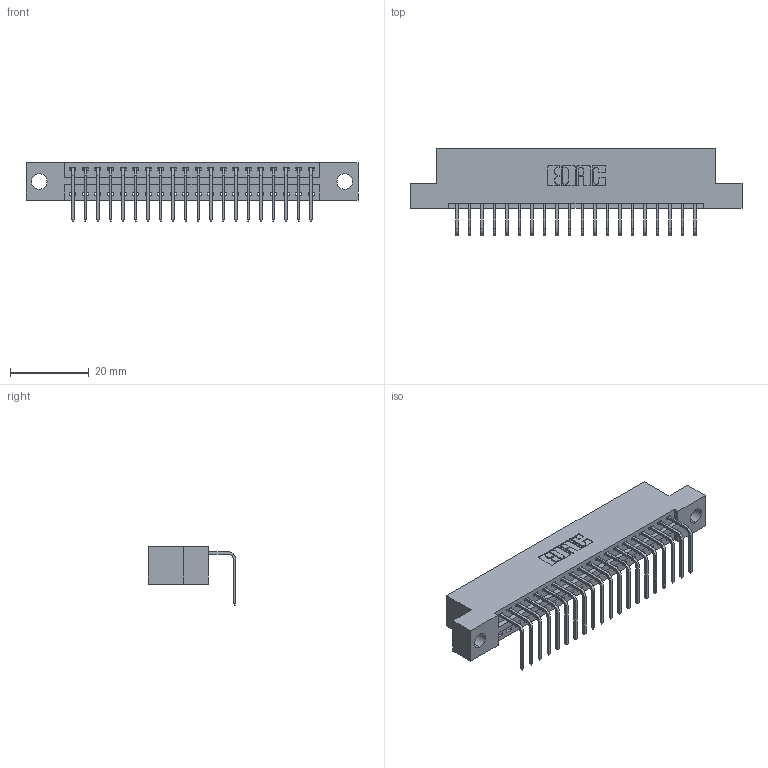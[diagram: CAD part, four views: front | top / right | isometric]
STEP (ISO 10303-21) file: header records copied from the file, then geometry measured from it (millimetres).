
FILE_DESCRIPTION (( 'STEP AP203' ), '1' );
FILE_NAME ('346-020-558-104.STEP', '2022-05-05T17:06:06', ( '' ), ( '' ), 'SwSTEP 2.0', 'SolidWorks 2020', '' );
FILE_SCHEMA (( 'CONFIG_CONTROL_DESIGN' ));
Length unit declared in the file: inch
Products named in the file (3): 346 Part_Flush Mounting Lugs - 0.156 Dia-TH; 346-020-558-104; 345-292-001_558 Tail - 2
Assembly tree (21 placements, depth 2):
  346-020-558-104
    346 Part_Flush Mounting Lugs - 0.156 Dia-TH
    345-292-001_558 Tail - 2  x20
Bounding box: 84.07 x 22.16 x 14.73 mm (x, y, z)
Volume: 7856.9 mm3; surface area: 9817.4 mm2
Topology: 21 solids, 21 shells, 1336 faces, 4005 edges, 2642 vertices
Faces by surface type: plane 930, cylinder 406
Entity records: 15877 total; most frequent: CARTESIAN_POINT 2738, ORIENTED_EDGE 2690, DIRECTION 2441, EDGE_CURVE 1345, LINE 1133, VECTOR 1133, VERTEX_POINT 894, AXIS2_PLACEMENT_3D 654
